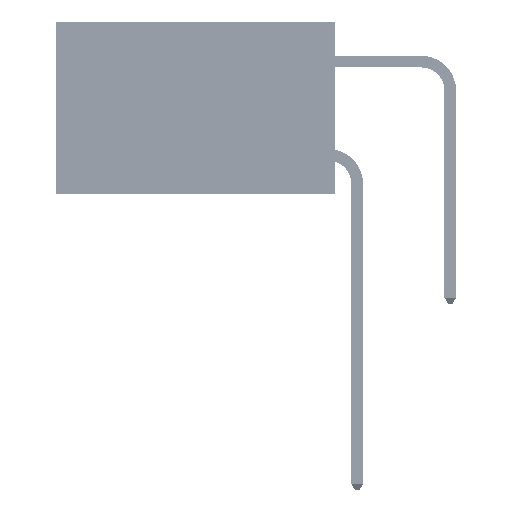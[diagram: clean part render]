
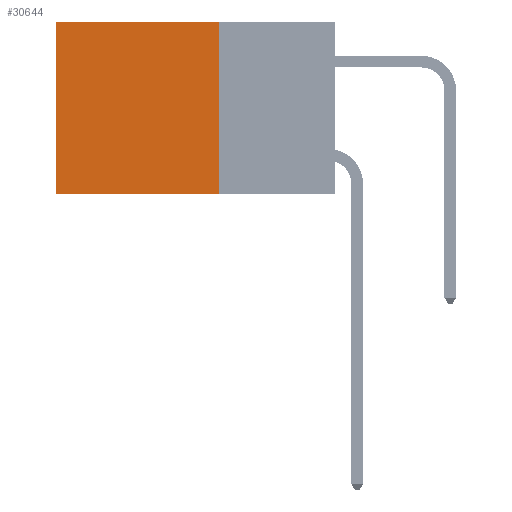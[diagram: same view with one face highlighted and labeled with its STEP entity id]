
A CAD part, left-side view. The second image highlights one B-rep face of the part: STEP entity #30644.
In plain terms, the highlighted planar face has unit normal (-1, 0, 0).
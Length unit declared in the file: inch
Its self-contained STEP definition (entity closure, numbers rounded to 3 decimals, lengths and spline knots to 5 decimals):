
#386 = EDGE_CURVE ( 'NONE', #38974, #45396, #46320, .T. ) ;
#2518 = DIRECTION ( 'NONE',  ( 1., 0., 0. ) ) ;
#3642 = CARTESIAN_POINT ( 'NONE',  ( 0.2875, 0.25, -0.37 ) ) ;
#6480 = FACE_OUTER_BOUND ( 'NONE', #34011, .T. ) ;
#7102 = DIRECTION ( 'NONE',  ( 0., 1., 0. ) ) ;
#7368 = LINE ( 'NONE', #3642, #24921 ) ;
#9654 = LINE ( 'NONE', #10707, #36655 ) ;
#10289 = VERTEX_POINT ( 'NONE', #39549 ) ;
#10707 = CARTESIAN_POINT ( 'NONE',  ( 0.2875, 0.6, 0. ) ) ;
#11179 = CARTESIAN_POINT ( 'NONE',  ( 0.2875, 0.25, 0. ) ) ;
#12385 = EDGE_CURVE ( 'NONE', #38974, #35302, #15780, .T. ) ;
#13082 = VECTOR ( 'NONE', #30795, 39.37008 ) ;
#13171 = CARTESIAN_POINT ( 'NONE',  ( 0.2875, 0.6, 0. ) ) ;
#15780 = LINE ( 'NONE', #48381, #29814 ) ;
#18607 = DIRECTION ( 'NONE',  ( 0., 0., -1. ) ) ;
#19328 = ORIENTED_EDGE ( 'NONE', *, *, #45595, .F. ) ;
#22563 = PLANE ( 'NONE',  #36953 ) ;
#23941 = DIRECTION ( 'NONE',  ( 0., 0., -1. ) ) ;
#24921 = VECTOR ( 'NONE', #7102, 39.37008 ) ;
#25575 = ORIENTED_EDGE ( 'NONE', *, *, #12385, .F. ) ;
#25600 = ORIENTED_EDGE ( 'NONE', *, *, #36227, .T. ) ;
#29814 = VECTOR ( 'NONE', #23941, 39.37008 ) ;
#30644 = ADVANCED_FACE ( 'NONE', ( #6480 ), #22563, .F. ) ;
#30795 = DIRECTION ( 'NONE',  ( 0., 1., 0. ) ) ;
#33266 = CARTESIAN_POINT ( 'NONE',  ( 0.2875, 0.25, -0.37 ) ) ;
#34011 = EDGE_LOOP ( 'NONE', ( #25600, #19328, #25575, #35633 ) ) ;
#35302 = VERTEX_POINT ( 'NONE', #33266 ) ;
#35633 = ORIENTED_EDGE ( 'NONE', *, *, #386, .T. ) ;
#36227 = EDGE_CURVE ( 'NONE', #45396, #10289, #9654, .T. ) ;
#36655 = VECTOR ( 'NONE', #18607, 39.37008 ) ;
#36953 = AXIS2_PLACEMENT_3D ( 'NONE', #38589, #2518, #46755 ) ;
#38589 = CARTESIAN_POINT ( 'NONE',  ( 0.2875, 0.25, 0. ) ) ;
#38974 = VERTEX_POINT ( 'NONE', #11179 ) ;
#39549 = CARTESIAN_POINT ( 'NONE',  ( 0.2875, 0.6, -0.37 ) ) ;
#45396 = VERTEX_POINT ( 'NONE', #13171 ) ;
#45595 = EDGE_CURVE ( 'NONE', #35302, #10289, #7368, .T. ) ;
#46320 = LINE ( 'NONE', #50779, #13082 ) ;
#46755 = DIRECTION ( 'NONE',  ( 0., 0., -1. ) ) ;
#48381 = CARTESIAN_POINT ( 'NONE',  ( 0.2875, 0.25, 0. ) ) ;
#50779 = CARTESIAN_POINT ( 'NONE',  ( 0.2875, 0.25, 0. ) ) ;
